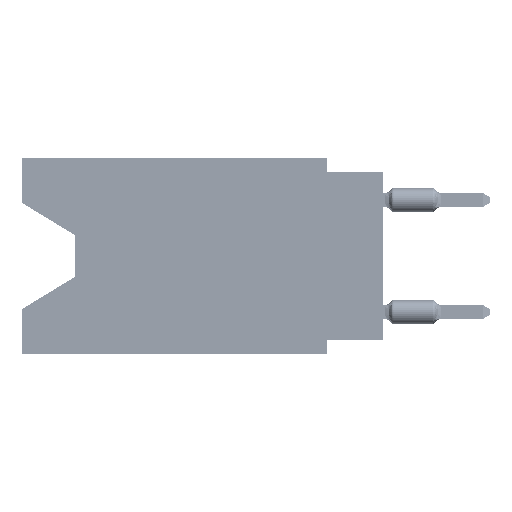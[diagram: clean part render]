
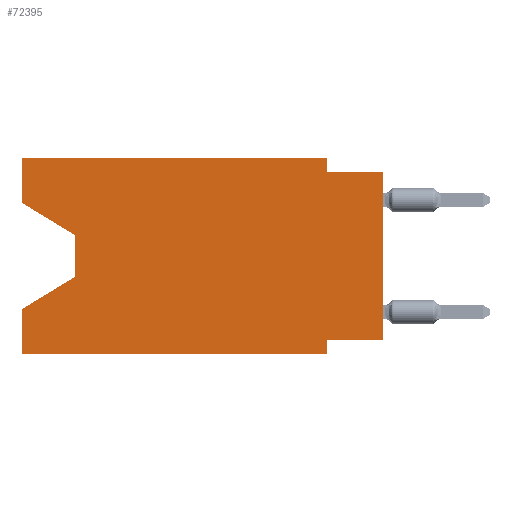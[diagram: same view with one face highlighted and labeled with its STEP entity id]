
A CAD part, left-side view. The second image highlights one B-rep face of the part: STEP entity #72395.
In plain terms, the highlighted planar face has unit normal (-1, 0, 0).
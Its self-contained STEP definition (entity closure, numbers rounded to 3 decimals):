
#906 = DIRECTION ( 'NONE',  ( 0., -1., 0. ) ) ;
#2039 = VERTEX_POINT ( 'NONE', #11712 ) ;
#4569 = DIRECTION ( 'NONE',  ( 0., 0., -1. ) ) ;
#4825 = VECTOR ( 'NONE', #906, 1000. ) ;
#6535 = ORIENTED_EDGE ( 'NONE', *, *, #59624, .F. ) ;
#9993 = LINE ( 'NONE', #38111, #36176 ) ;
#10165 = LINE ( 'NONE', #40786, #35152 ) ;
#11481 = CARTESIAN_POINT ( 'NONE',  ( 0., 0., 0. ) ) ;
#11712 = CARTESIAN_POINT ( 'NONE',  ( 0., 13.97, -3.505 ) ) ;
#11926 = EDGE_CURVE ( 'NONE', #64344, #24255, #10165, .T. ) ;
#12014 = VECTOR ( 'NONE', #57717, 1000. ) ;
#12366 = ORIENTED_EDGE ( 'NONE', *, *, #47703, .T. ) ;
#13527 = EDGE_CURVE ( 'NONE', #32196, #68156, #30970, .T. ) ;
#14342 = VECTOR ( 'NONE', #4569, 1000. ) ;
#15048 = EDGE_CURVE ( 'NONE', #54784, #18001, #46687, .T. ) ;
#15837 = VERTEX_POINT ( 'NONE', #39677 ) ;
#16039 = DIRECTION ( 'NONE',  ( 0., 0., -1. ) ) ;
#16200 = CARTESIAN_POINT ( 'NONE',  ( 0., 13.97, -3.505 ) ) ;
#16991 = CARTESIAN_POINT ( 'NONE',  ( 0., 2.54, -0.635 ) ) ;
#17948 = VECTOR ( 'NONE', #45269, 1000. ) ;
#18001 = VERTEX_POINT ( 'NONE', #51550 ) ;
#18633 = CARTESIAN_POINT ( 'NONE',  ( 0., 2.54, 0. ) ) ;
#20490 = VECTOR ( 'NONE', #65816, 1000. ) ;
#20562 = PLANE ( 'NONE',  #56669 ) ;
#21066 = CARTESIAN_POINT ( 'NONE',  ( 0., 2.54, -8.89 ) ) ;
#21139 = VECTOR ( 'NONE', #57223, 1000. ) ;
#22031 = LINE ( 'NONE', #73766, #42049 ) ;
#23859 = EDGE_CURVE ( 'NONE', #31990, #73511, #51212, .T. ) ;
#24115 = ORIENTED_EDGE ( 'NONE', *, *, #15048, .F. ) ;
#24177 = DIRECTION ( 'NONE',  ( 0., 0., 1. ) ) ;
#24255 = VERTEX_POINT ( 'NONE', #61615 ) ;
#24924 = LINE ( 'NONE', #65021, #4825 ) ;
#28790 = DIRECTION ( 'NONE',  ( 0., 0., 1. ) ) ;
#29578 = CARTESIAN_POINT ( 'NONE',  ( 0., 16.383, 0. ) ) ;
#30238 = VECTOR ( 'NONE', #24177, 1000. ) ;
#30970 = LINE ( 'NONE', #59471, #20490 ) ;
#31004 = ORIENTED_EDGE ( 'NONE', *, *, #23859, .F. ) ;
#31990 = VERTEX_POINT ( 'NONE', #18633 ) ;
#32196 = VERTEX_POINT ( 'NONE', #71088 ) ;
#33326 = ORIENTED_EDGE ( 'NONE', *, *, #61066, .F. ) ;
#34712 = EDGE_CURVE ( 'NONE', #2039, #15837, #38318, .T. ) ;
#35152 = VECTOR ( 'NONE', #28790, 1000. ) ;
#36176 = VECTOR ( 'NONE', #43377, 1000. ) ;
#36495 = CARTESIAN_POINT ( 'NONE',  ( 0., 16.383, -2.038 ) ) ;
#37156 = ORIENTED_EDGE ( 'NONE', *, *, #34712, .T. ) ;
#37642 = EDGE_CURVE ( 'NONE', #64344, #72289, #9993, .T. ) ;
#37860 = ORIENTED_EDGE ( 'NONE', *, *, #71726, .F. ) ;
#38111 = CARTESIAN_POINT ( 'NONE',  ( 0., 16.383, -8.89 ) ) ;
#38318 = LINE ( 'NONE', #16200, #14342 ) ;
#39677 = CARTESIAN_POINT ( 'NONE',  ( 0., 13.97, -5.385 ) ) ;
#40786 = CARTESIAN_POINT ( 'NONE',  ( 0., 16.383, 0. ) ) ;
#41198 = CARTESIAN_POINT ( 'NONE',  ( 0., 2.54, -8.255 ) ) ;
#42010 = CARTESIAN_POINT ( 'NONE',  ( 0., 13.97, -5.385 ) ) ;
#42049 = VECTOR ( 'NONE', #16039, 1000. ) ;
#43377 = DIRECTION ( 'NONE',  ( 0., -1., 0. ) ) ;
#43438 = DIRECTION ( 'NONE',  ( 1., 0., 0. ) ) ;
#45269 = DIRECTION ( 'NONE',  ( 0., -0.855, -0.519 ) ) ;
#45856 = VERTEX_POINT ( 'NONE', #47631 ) ;
#45864 = EDGE_CURVE ( 'NONE', #15837, #24255, #47265, .T. ) ;
#46687 = LINE ( 'NONE', #74073, #30238 ) ;
#47265 = LINE ( 'NONE', #42010, #55680 ) ;
#47631 = CARTESIAN_POINT ( 'NONE',  ( 0., 0., -0.635 ) ) ;
#47703 = EDGE_CURVE ( 'NONE', #32196, #45856, #51240, .T. ) ;
#47910 = ORIENTED_EDGE ( 'NONE', *, *, #13527, .F. ) ;
#51212 = LINE ( 'NONE', #68808, #62099 ) ;
#51240 = LINE ( 'NONE', #11481, #21139 ) ;
#51550 = CARTESIAN_POINT ( 'NONE',  ( 0., 16.383, 0. ) ) ;
#54784 = VERTEX_POINT ( 'NONE', #36495 ) ;
#55388 = LINE ( 'NONE', #67744, #17948 ) ;
#55680 = VECTOR ( 'NONE', #59602, 1000. ) ;
#56071 = ORIENTED_EDGE ( 'NONE', *, *, #37642, .T. ) ;
#56255 = ORIENTED_EDGE ( 'NONE', *, *, #11926, .F. ) ;
#56669 = AXIS2_PLACEMENT_3D ( 'NONE', #65924, #43438, #60677 ) ;
#57223 = DIRECTION ( 'NONE',  ( 0., 0., 1. ) ) ;
#57717 = DIRECTION ( 'NONE',  ( 0., -1., 0. ) ) ;
#59471 = CARTESIAN_POINT ( 'NONE',  ( 0., 0., -8.255 ) ) ;
#59602 = DIRECTION ( 'NONE',  ( 0., 0.855, -0.519 ) ) ;
#59624 = EDGE_CURVE ( 'NONE', #18001, #31990, #63334, .T. ) ;
#60677 = DIRECTION ( 'NONE',  ( 0., 0., -1. ) ) ;
#61066 = EDGE_CURVE ( 'NONE', #73511, #45856, #24924, .T. ) ;
#61615 = CARTESIAN_POINT ( 'NONE',  ( 0., 16.383, -6.852 ) ) ;
#62099 = VECTOR ( 'NONE', #73692, 1000. ) ;
#63302 = EDGE_LOOP ( 'NONE', ( #70379, #37156, #67291, #56255, #56071, #37860, #47910, #12366, #33326, #31004, #6535, #24115 ) ) ;
#63334 = LINE ( 'NONE', #29578, #12014 ) ;
#64344 = VERTEX_POINT ( 'NONE', #72661 ) ;
#65021 = CARTESIAN_POINT ( 'NONE',  ( 0., 0., -0.635 ) ) ;
#65691 = FACE_OUTER_BOUND ( 'NONE', #63302, .T. ) ;
#65816 = DIRECTION ( 'NONE',  ( 0., 1., 0. ) ) ;
#65924 = CARTESIAN_POINT ( 'NONE',  ( 0., 16.383, 0. ) ) ;
#67291 = ORIENTED_EDGE ( 'NONE', *, *, #45864, .T. ) ;
#67744 = CARTESIAN_POINT ( 'NONE',  ( 0., 16.383, -2.038 ) ) ;
#68156 = VERTEX_POINT ( 'NONE', #41198 ) ;
#68355 = EDGE_CURVE ( 'NONE', #54784, #2039, #55388, .T. ) ;
#68808 = CARTESIAN_POINT ( 'NONE',  ( 0., 2.54, 0. ) ) ;
#70379 = ORIENTED_EDGE ( 'NONE', *, *, #68355, .T. ) ;
#71088 = CARTESIAN_POINT ( 'NONE',  ( 0., 0., -8.255 ) ) ;
#71726 = EDGE_CURVE ( 'NONE', #68156, #72289, #22031, .T. ) ;
#72289 = VERTEX_POINT ( 'NONE', #21066 ) ;
#72395 = ADVANCED_FACE ( 'NONE', ( #65691 ), #20562, .F. ) ;
#72661 = CARTESIAN_POINT ( 'NONE',  ( 0., 16.383, -8.89 ) ) ;
#73511 = VERTEX_POINT ( 'NONE', #16991 ) ;
#73692 = DIRECTION ( 'NONE',  ( 0., 0., -1. ) ) ;
#73766 = CARTESIAN_POINT ( 'NONE',  ( 0., 2.54, -8.89 ) ) ;
#74073 = CARTESIAN_POINT ( 'NONE',  ( 0., 16.383, 0. ) ) ;
